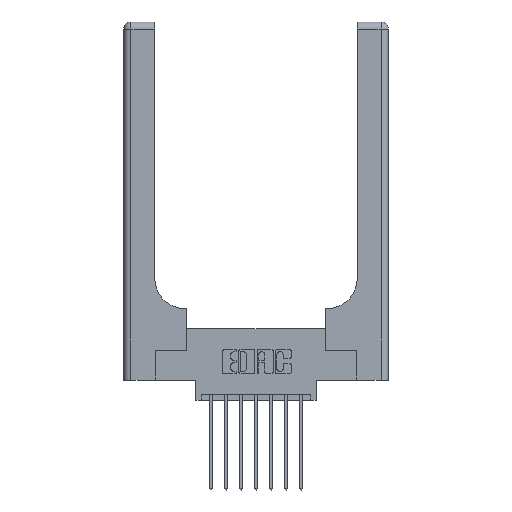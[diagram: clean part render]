
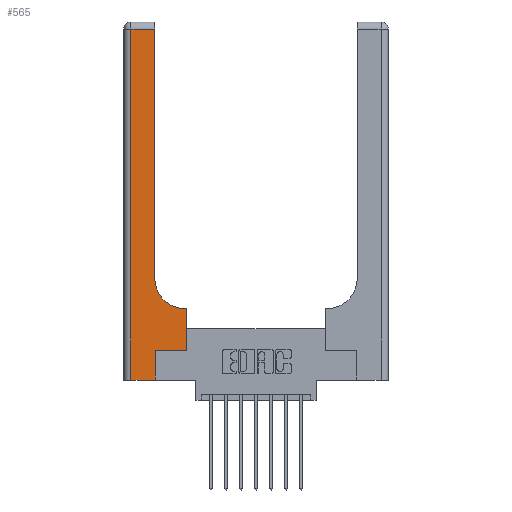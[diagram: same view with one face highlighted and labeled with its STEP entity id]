
A CAD part, top view. The second image highlights one B-rep face of the part: STEP entity #565.
In plain terms, the highlighted planar face has unit normal (0, 0, 1).
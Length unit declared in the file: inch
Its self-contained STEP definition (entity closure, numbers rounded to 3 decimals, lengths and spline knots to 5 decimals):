
#53 = DIRECTION ( 'NONE',  ( 0., 0., -1. ) ) ;
#149 = VERTEX_POINT ( 'NONE', #5857 ) ;
#341 = CARTESIAN_POINT ( 'NONE',  ( 0.265, 0., 0.37 ) ) ;
#431 = CARTESIAN_POINT ( 'NONE',  ( 0.265, 0., 0.37 ) ) ;
#550 = DIRECTION ( 'NONE',  ( 0., 0., -1. ) ) ;
#565 = ADVANCED_FACE ( 'NONE', ( #6828 ), #2345, .F. ) ;
#689 = CARTESIAN_POINT ( 'NONE',  ( 0.26, 0.85, 0.37 ) ) ;
#700 = EDGE_CURVE ( 'NONE', #8835, #13157, #10773, .T. ) ;
#860 = AXIS2_PLACEMENT_3D ( 'NONE', #14497, #550, #7404 ) ;
#943 = ORIENTED_EDGE ( 'NONE', *, *, #6799, .T. ) ;
#1148 = VECTOR ( 'NONE', #2386, 39.37008 ) ;
#1339 = CIRCLE ( 'NONE', #860, 0.25 ) ;
#1496 = CARTESIAN_POINT ( 'NONE',  ( 0., 0., 0.37 ) ) ;
#1563 = EDGE_CURVE ( 'NONE', #9369, #6317, #7298, .T. ) ;
#1659 = EDGE_CURVE ( 'NONE', #13157, #3394, #1900, .T. ) ;
#1775 = VECTOR ( 'NONE', #13751, 39.37008 ) ;
#1900 = LINE ( 'NONE', #8796, #9662 ) ;
#1975 = DIRECTION ( 'NONE',  ( 1., 0., 0. ) ) ;
#2345 = PLANE ( 'NONE',  #12909 ) ;
#2386 = DIRECTION ( 'NONE',  ( 0., 1., 0. ) ) ;
#2787 = DIRECTION ( 'NONE',  ( 1., 0., 0. ) ) ;
#3171 = VECTOR ( 'NONE', #2787, 39.37008 ) ;
#3394 = VERTEX_POINT ( 'NONE', #4741 ) ;
#3803 = CARTESIAN_POINT ( 'NONE',  ( 0.26, 0.6, 0.37 ) ) ;
#3981 = VERTEX_POINT ( 'NONE', #689 ) ;
#3984 = CARTESIAN_POINT ( 'NONE',  ( 0.51, 0.6, 0.37 ) ) ;
#4692 = DIRECTION ( 'NONE',  ( -1., 0., 0. ) ) ;
#4734 = LINE ( 'NONE', #6105, #9283 ) ;
#4741 = CARTESIAN_POINT ( 'NONE',  ( 0.528, 0.25, 0.37 ) ) ;
#5282 = ORIENTED_EDGE ( 'NONE', *, *, #700, .T. ) ;
#5388 = EDGE_LOOP ( 'NONE', ( #14066, #12812, #9057, #9563, #5282, #8301, #943, #8536, #12168 ) ) ;
#5857 = CARTESIAN_POINT ( 'NONE',  ( 0.26, 2.94, 0.37 ) ) ;
#6056 = VECTOR ( 'NONE', #8624, 39.37008 ) ;
#6105 = CARTESIAN_POINT ( 'NONE',  ( 0.06, 3., 0.37 ) ) ;
#6317 = VERTEX_POINT ( 'NONE', #3984 ) ;
#6321 = EDGE_CURVE ( 'NONE', #6317, #3981, #1339, .T. ) ;
#6668 = LINE ( 'NONE', #10392, #1775 ) ;
#6799 = EDGE_CURVE ( 'NONE', #3394, #9369, #8082, .T. ) ;
#6828 = FACE_OUTER_BOUND ( 'NONE', #5388, .T. ) ;
#7298 = LINE ( 'NONE', #3803, #14292 ) ;
#7310 = EDGE_CURVE ( 'NONE', #149, #12208, #11430, .T. ) ;
#7404 = DIRECTION ( 'NONE',  ( 1., 0., 0. ) ) ;
#7491 = CARTESIAN_POINT ( 'NONE',  ( 0.265, 0.25, 0.37 ) ) ;
#8000 = DIRECTION ( 'NONE',  ( -1., 0., 0. ) ) ;
#8082 = LINE ( 'NONE', #9222, #1148 ) ;
#8239 = DIRECTION ( 'NONE',  ( 0., -1., 0. ) ) ;
#8301 = ORIENTED_EDGE ( 'NONE', *, *, #1659, .T. ) ;
#8508 = DIRECTION ( 'NONE',  ( -1., 0., 0. ) ) ;
#8536 = ORIENTED_EDGE ( 'NONE', *, *, #1563, .T. ) ;
#8544 = CARTESIAN_POINT ( 'NONE',  ( 0.528, 0.6, 0.37 ) ) ;
#8624 = DIRECTION ( 'NONE',  ( 0., 1., 0. ) ) ;
#8796 = CARTESIAN_POINT ( 'NONE',  ( 0.265, 0.25, 0.37 ) ) ;
#8835 = VERTEX_POINT ( 'NONE', #431 ) ;
#9057 = ORIENTED_EDGE ( 'NONE', *, *, #11656, .T. ) ;
#9093 = EDGE_CURVE ( 'NONE', #3981, #149, #6668, .T. ) ;
#9222 = CARTESIAN_POINT ( 'NONE',  ( 0.528, 0.25, 0.37 ) ) ;
#9276 = CARTESIAN_POINT ( 'NONE',  ( 0., 2.94, 0.37 ) ) ;
#9283 = VECTOR ( 'NONE', #8239, 39.37008 ) ;
#9369 = VERTEX_POINT ( 'NONE', #8544 ) ;
#9563 = ORIENTED_EDGE ( 'NONE', *, *, #11441, .T. ) ;
#9662 = VECTOR ( 'NONE', #1975, 39.37008 ) ;
#10392 = CARTESIAN_POINT ( 'NONE',  ( 0.26, 3., 0.37 ) ) ;
#10688 = CARTESIAN_POINT ( 'NONE',  ( 0.06, 0., 0.37 ) ) ;
#10773 = LINE ( 'NONE', #341, #6056 ) ;
#10889 = VECTOR ( 'NONE', #8000, 39.37008 ) ;
#11430 = LINE ( 'NONE', #9276, #10889 ) ;
#11441 = EDGE_CURVE ( 'NONE', #13139, #8835, #14294, .T. ) ;
#11477 = CARTESIAN_POINT ( 'NONE',  ( 0., 3., 0.37 ) ) ;
#11656 = EDGE_CURVE ( 'NONE', #12208, #13139, #4734, .T. ) ;
#12168 = ORIENTED_EDGE ( 'NONE', *, *, #6321, .T. ) ;
#12208 = VERTEX_POINT ( 'NONE', #12248 ) ;
#12248 = CARTESIAN_POINT ( 'NONE',  ( 0.06, 2.94, 0.37 ) ) ;
#12812 = ORIENTED_EDGE ( 'NONE', *, *, #7310, .T. ) ;
#12909 = AXIS2_PLACEMENT_3D ( 'NONE', #11477, #53, #4692 ) ;
#13139 = VERTEX_POINT ( 'NONE', #10688 ) ;
#13157 = VERTEX_POINT ( 'NONE', #7491 ) ;
#13751 = DIRECTION ( 'NONE',  ( 0., 1., 0. ) ) ;
#14066 = ORIENTED_EDGE ( 'NONE', *, *, #9093, .T. ) ;
#14292 = VECTOR ( 'NONE', #8508, 39.37008 ) ;
#14294 = LINE ( 'NONE', #1496, #3171 ) ;
#14497 = CARTESIAN_POINT ( 'NONE',  ( 0.51, 0.85, 0.37 ) ) ;
